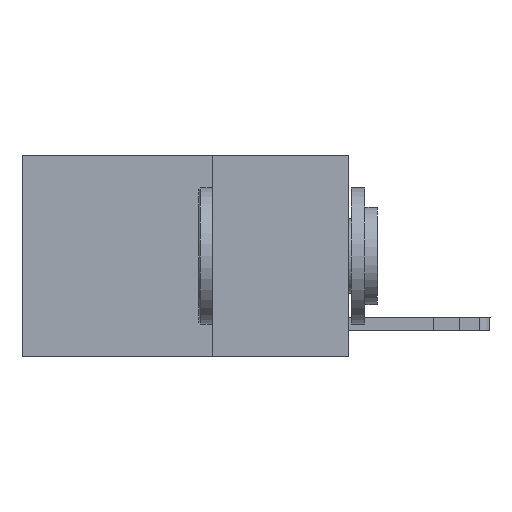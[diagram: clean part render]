
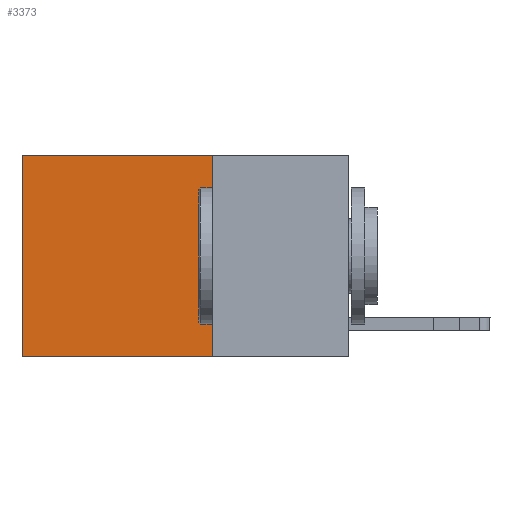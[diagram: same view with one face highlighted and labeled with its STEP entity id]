
A CAD part, left-side view. The second image highlights one B-rep face of the part: STEP entity #3373.
In plain terms, the highlighted planar face has unit normal (-1, 0, 0).
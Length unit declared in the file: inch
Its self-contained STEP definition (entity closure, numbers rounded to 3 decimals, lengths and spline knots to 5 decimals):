
#197 = EDGE_CURVE ( 'NONE', #14142, #2122, #4974, .T. ) ;
#1175 = DIRECTION ( 'NONE',  ( 1., 0., 0. ) ) ;
#1411 = VECTOR ( 'NONE', #1603, 39.37008 ) ;
#1521 = DIRECTION ( 'NONE',  ( 0., 1., 0. ) ) ;
#1551 = ORIENTED_EDGE ( 'NONE', *, *, #197, .F. ) ;
#1603 = DIRECTION ( 'NONE',  ( 0., 1., 0. ) ) ;
#1692 = ORIENTED_EDGE ( 'NONE', *, *, #4122, .F. ) ;
#2064 = EDGE_LOOP ( 'NONE', ( #9102, #1692, #1551, #3720 ) ) ;
#2122 = VERTEX_POINT ( 'NONE', #11630 ) ;
#2239 = EDGE_CURVE ( 'NONE', #10734, #12648, #5033, .T. ) ;
#2415 = FACE_OUTER_BOUND ( 'NONE', #2064, .T. ) ;
#2677 = LINE ( 'NONE', #7151, #2786 ) ;
#2786 = VECTOR ( 'NONE', #1521, 39.37008 ) ;
#3373 = ADVANCED_FACE ( 'NONE', ( #2415 ), #6968, .F. ) ;
#3720 = ORIENTED_EDGE ( 'NONE', *, *, #6737, .T. ) ;
#4122 = EDGE_CURVE ( 'NONE', #2122, #12648, #6261, .T. ) ;
#4129 = AXIS2_PLACEMENT_3D ( 'NONE', #9277, #1175, #14922 ) ;
#4222 = CARTESIAN_POINT ( 'NONE',  ( 0.2625, 0.6, -0.37 ) ) ;
#4974 = LINE ( 'NONE', #11558, #6195 ) ;
#5033 = LINE ( 'NONE', #9502, #12294 ) ;
#6195 = VECTOR ( 'NONE', #10412, 39.37008 ) ;
#6261 = LINE ( 'NONE', #6398, #1411 ) ;
#6398 = CARTESIAN_POINT ( 'NONE',  ( 0.2625, 0.25, -0.37 ) ) ;
#6737 = EDGE_CURVE ( 'NONE', #14142, #10734, #2677, .T. ) ;
#6968 = PLANE ( 'NONE',  #4129 ) ;
#7151 = CARTESIAN_POINT ( 'NONE',  ( 0.2625, 0.25, 0. ) ) ;
#8418 = CARTESIAN_POINT ( 'NONE',  ( 0.2625, 0.25, 0. ) ) ;
#8480 = CARTESIAN_POINT ( 'NONE',  ( 0.2625, 0.6, 0. ) ) ;
#9102 = ORIENTED_EDGE ( 'NONE', *, *, #2239, .T. ) ;
#9277 = CARTESIAN_POINT ( 'NONE',  ( 0.2625, 0.25, 0. ) ) ;
#9502 = CARTESIAN_POINT ( 'NONE',  ( 0.2625, 0.6, 0. ) ) ;
#10412 = DIRECTION ( 'NONE',  ( 0., 0., -1. ) ) ;
#10734 = VERTEX_POINT ( 'NONE', #8480 ) ;
#11558 = CARTESIAN_POINT ( 'NONE',  ( 0.2625, 0.25, 0. ) ) ;
#11630 = CARTESIAN_POINT ( 'NONE',  ( 0.2625, 0.25, -0.37 ) ) ;
#12294 = VECTOR ( 'NONE', #12871, 39.37008 ) ;
#12648 = VERTEX_POINT ( 'NONE', #4222 ) ;
#12871 = DIRECTION ( 'NONE',  ( 0., 0., -1. ) ) ;
#14142 = VERTEX_POINT ( 'NONE', #8418 ) ;
#14922 = DIRECTION ( 'NONE',  ( 0., 0., -1. ) ) ;
